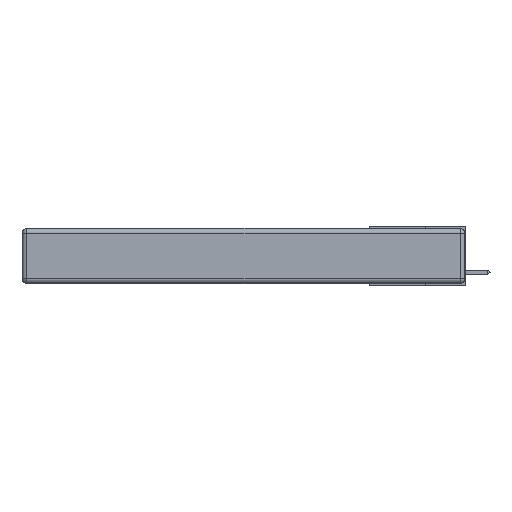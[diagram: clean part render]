
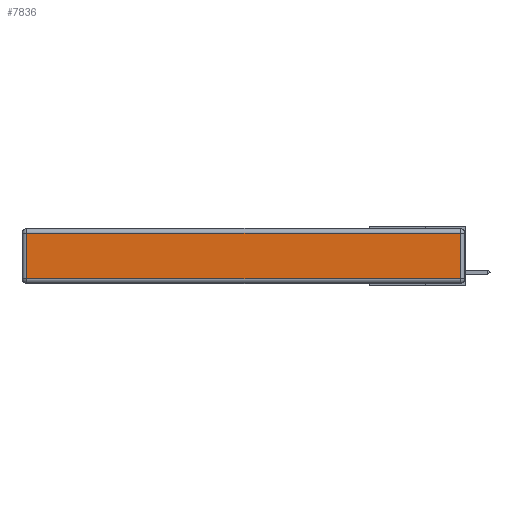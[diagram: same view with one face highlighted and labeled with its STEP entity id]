
A CAD part, left-side view. The second image highlights one B-rep face of the part: STEP entity #7836.
In plain terms, the highlighted planar face has unit normal (-1, 0, 0).
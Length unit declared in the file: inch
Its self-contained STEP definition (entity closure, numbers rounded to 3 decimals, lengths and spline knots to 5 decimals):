
#627 = CARTESIAN_POINT ( 'NONE',  ( 0., 2.72, -0.313 ) ) ;
#713 = DIRECTION ( 'NONE',  ( -1., 0., 0. ) ) ;
#891 = VECTOR ( 'NONE', #8548, 39.37008 ) ;
#1336 = ORIENTED_EDGE ( 'NONE', *, *, #2416, .T. ) ;
#1803 = DIRECTION ( 'NONE',  ( 0., -1., 0. ) ) ;
#2017 = VECTOR ( 'NONE', #31775, 39.37008 ) ;
#2416 = EDGE_CURVE ( 'NONE', #2957, #15580, #21256, .T. ) ;
#2957 = VERTEX_POINT ( 'NONE', #3660 ) ;
#3660 = CARTESIAN_POINT ( 'NONE',  ( 0., 2.72, -0.03 ) ) ;
#3670 = LINE ( 'NONE', #6345, #29031 ) ;
#4352 = CARTESIAN_POINT ( 'NONE',  ( 0., 2.72, -0.343 ) ) ;
#4739 = ORIENTED_EDGE ( 'NONE', *, *, #26632, .T. ) ;
#5786 = DIRECTION ( 'NONE',  ( 0., 0., 1. ) ) ;
#6345 = CARTESIAN_POINT ( 'NONE',  ( 0., 0., -0.313 ) ) ;
#6491 = VERTEX_POINT ( 'NONE', #24182 ) ;
#7836 = ADVANCED_FACE ( 'NONE', ( #24396 ), #8049, .T. ) ;
#8049 = PLANE ( 'NONE',  #28124 ) ;
#8548 = DIRECTION ( 'NONE',  ( 0., 1., 0. ) ) ;
#9613 = ORIENTED_EDGE ( 'NONE', *, *, #26961, .T. ) ;
#10406 = LINE ( 'NONE', #21640, #2017 ) ;
#10696 = CARTESIAN_POINT ( 'NONE',  ( 0., 2.75, -0.03 ) ) ;
#15580 = VERTEX_POINT ( 'NONE', #627 ) ;
#20463 = VECTOR ( 'NONE', #21767, 39.37008 ) ;
#21256 = LINE ( 'NONE', #4352, #20463 ) ;
#21640 = CARTESIAN_POINT ( 'NONE',  ( 0., 0.03, -0.343 ) ) ;
#21767 = DIRECTION ( 'NONE',  ( 0., 0., -1. ) ) ;
#21888 = VERTEX_POINT ( 'NONE', #30606 ) ;
#22685 = EDGE_CURVE ( 'NONE', #15580, #6491, #3670, .T. ) ;
#23502 = EDGE_LOOP ( 'NONE', ( #28936, #4739, #9613, #1336 ) ) ;
#24182 = CARTESIAN_POINT ( 'NONE',  ( 0., 0.03, -0.313 ) ) ;
#24396 = FACE_OUTER_BOUND ( 'NONE', #23502, .T. ) ;
#25449 = LINE ( 'NONE', #10696, #891 ) ;
#25743 = CARTESIAN_POINT ( 'NONE',  ( 0., 0., -0.343 ) ) ;
#26632 = EDGE_CURVE ( 'NONE', #6491, #21888, #10406, .T. ) ;
#26961 = EDGE_CURVE ( 'NONE', #21888, #2957, #25449, .T. ) ;
#28124 = AXIS2_PLACEMENT_3D ( 'NONE', #25743, #713, #5786 ) ;
#28936 = ORIENTED_EDGE ( 'NONE', *, *, #22685, .T. ) ;
#29031 = VECTOR ( 'NONE', #1803, 39.37008 ) ;
#30606 = CARTESIAN_POINT ( 'NONE',  ( 0., 0.03, -0.03 ) ) ;
#31775 = DIRECTION ( 'NONE',  ( 0., 0., 1. ) ) ;
